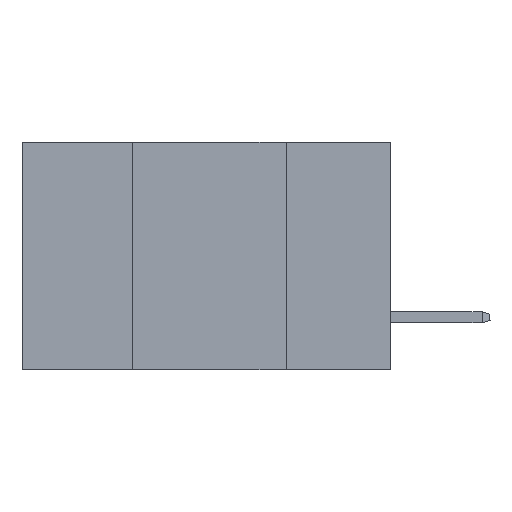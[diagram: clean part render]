
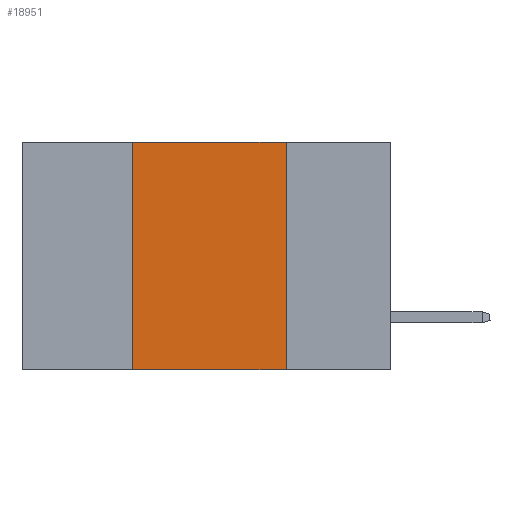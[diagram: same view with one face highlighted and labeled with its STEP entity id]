
A CAD part, left-side view. The second image highlights one B-rep face of the part: STEP entity #18951.
In plain terms, the highlighted planar face has unit normal (-1, 0, 0).
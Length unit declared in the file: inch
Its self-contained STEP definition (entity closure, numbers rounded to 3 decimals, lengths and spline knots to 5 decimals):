
#2005 = VERTEX_POINT ( 'NONE', #25441 ) ;
#2874 = DIRECTION ( 'NONE',  ( 0., -1., 0. ) ) ;
#3676 = EDGE_CURVE ( 'NONE', #10528, #2005, #38616, .T. ) ;
#5542 = AXIS2_PLACEMENT_3D ( 'NONE', #30927, #37605, #34178 ) ;
#6996 = VECTOR ( 'NONE', #17001, 39.37008 ) ;
#9988 = CARTESIAN_POINT ( 'NONE',  ( 0., 0.17, -0.37 ) ) ;
#10528 = VERTEX_POINT ( 'NONE', #40946 ) ;
#11170 = DIRECTION ( 'NONE',  ( 0., -1., 0. ) ) ;
#11637 = VECTOR ( 'NONE', #36703, 39.37008 ) ;
#14630 = LINE ( 'NONE', #17551, #11637 ) ;
#17001 = DIRECTION ( 'NONE',  ( 0., 0., -1. ) ) ;
#17353 = EDGE_LOOP ( 'NONE', ( #40058, #42056, #34669, #31694 ) ) ;
#17551 = CARTESIAN_POINT ( 'NONE',  ( 0., 0.42, 0. ) ) ;
#18729 = VECTOR ( 'NONE', #2874, 39.37008 ) ;
#18951 = ADVANCED_FACE ( 'NONE', ( #26065 ), #26792, .F. ) ;
#21302 = VECTOR ( 'NONE', #11170, 39.37008 ) ;
#21910 = EDGE_CURVE ( 'NONE', #37942, #24312, #29930, .T. ) ;
#24312 = VERTEX_POINT ( 'NONE', #9988 ) ;
#24358 = LINE ( 'NONE', #27761, #6996 ) ;
#25441 = CARTESIAN_POINT ( 'NONE',  ( 0., 0.17, 0. ) ) ;
#25650 = CARTESIAN_POINT ( 'NONE',  ( 0., 0.6, 0. ) ) ;
#26065 = FACE_OUTER_BOUND ( 'NONE', #17353, .T. ) ;
#26792 = PLANE ( 'NONE',  #5542 ) ;
#27761 = CARTESIAN_POINT ( 'NONE',  ( 0., 0.17, 0. ) ) ;
#29930 = LINE ( 'NONE', #39017, #21302 ) ;
#30927 = CARTESIAN_POINT ( 'NONE',  ( 0., 0.6, 0. ) ) ;
#31694 = ORIENTED_EDGE ( 'NONE', *, *, #21910, .T. ) ;
#34178 = DIRECTION ( 'NONE',  ( 0., 0., -1. ) ) ;
#34669 = ORIENTED_EDGE ( 'NONE', *, *, #35352, .F. ) ;
#35352 = EDGE_CURVE ( 'NONE', #37942, #10528, #14630, .T. ) ;
#35535 = EDGE_CURVE ( 'NONE', #2005, #24312, #24358, .T. ) ;
#36703 = DIRECTION ( 'NONE',  ( 0., 0., 1. ) ) ;
#37605 = DIRECTION ( 'NONE',  ( 1., 0., 0. ) ) ;
#37898 = CARTESIAN_POINT ( 'NONE',  ( 0., 0.42, -0.37 ) ) ;
#37942 = VERTEX_POINT ( 'NONE', #37898 ) ;
#38616 = LINE ( 'NONE', #25650, #18729 ) ;
#39017 = CARTESIAN_POINT ( 'NONE',  ( 0., 0.6, -0.37 ) ) ;
#40058 = ORIENTED_EDGE ( 'NONE', *, *, #35535, .F. ) ;
#40946 = CARTESIAN_POINT ( 'NONE',  ( 0., 0.42, 0. ) ) ;
#42056 = ORIENTED_EDGE ( 'NONE', *, *, #3676, .F. ) ;
